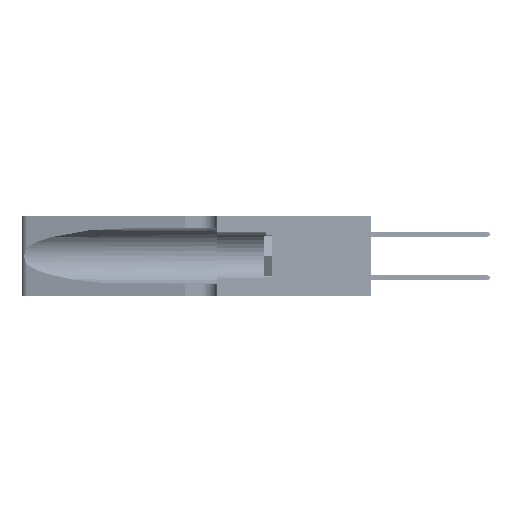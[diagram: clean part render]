
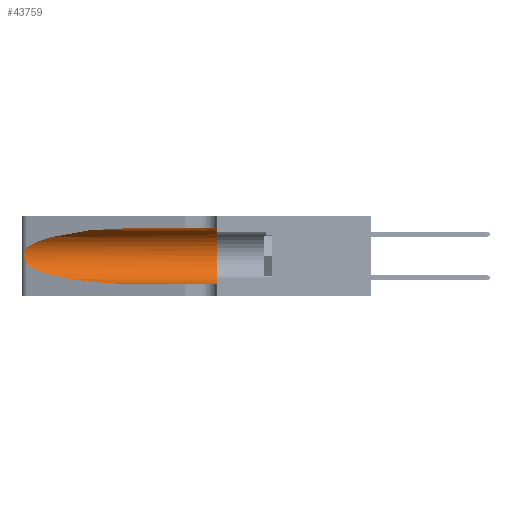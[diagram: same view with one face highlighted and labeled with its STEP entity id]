
A CAD part, left-side view. The second image highlights one B-rep face of the part: STEP entity #43759.
In plain terms, the highlighted cylindrical face has radius 3.308 mm (diameter 6.617 mm), a partial arc.
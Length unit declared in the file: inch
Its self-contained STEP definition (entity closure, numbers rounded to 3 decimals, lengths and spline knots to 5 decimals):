
#577 = CARTESIAN_POINT ( 'NONE',  ( 0.1305, 0.72297, 0.31525 ) ) ;
#794 = CARTESIAN_POINT ( 'NONE',  ( 0.25487, 1.22718, 0.22369 ) ) ;
#3253 = CARTESIAN_POINT ( 'NONE',  ( 0.18966, 0.96281, 0.31525 ) ) ;
#4161 = LINE ( 'NONE', #14341, #13640 ) ;
#4874 = CARTESIAN_POINT ( 'NONE',  ( 0.25854, 1.2359, 0.20912 ) ) ;
#5238 = ORIENTED_EDGE ( 'NONE', *, *, #36718, .T. ) ;
#5308 = ORIENTED_EDGE ( 'NONE', *, *, #21669, .T. ) ;
#6125 = DIRECTION ( 'NONE',  ( 0., -1., 0. ) ) ;
#7294 = CARTESIAN_POINT ( 'NONE',  ( 0.2373, 1.15595, 0.28018 ) ) ;
#8201 = VECTOR ( 'NONE', #6125, 39.37008 ) ;
#8937 = CARTESIAN_POINT ( 'NONE',  ( 0.26075, 1.23896, 0.19203 ) ) ;
#9291 = CARTESIAN_POINT ( 'NONE',  ( 0.25487, 1.22718, 0.22369 ) ) ;
#10169 = CARTESIAN_POINT ( 'NONE',  ( 0.1305, 1.61858, 0.185 ) ) ;
#11039 = EDGE_CURVE ( 'NONE', #23469, #43765, #18882, .T. ) ;
#12251 = DIRECTION ( 'NONE',  ( 0., 1., 0. ) ) ;
#12775 =( BOUNDED_CURVE ( )  B_SPLINE_CURVE ( 3, ( #29696, #41445, #13868, #41618 ),
 .UNSPECIFIED., .F., .F. ) 
 B_SPLINE_CURVE_WITH_KNOTS ( ( 4, 4 ),
 ( 3.44316, 4.71239 ),
 .UNSPECIFIED. ) 
 CURVE ( )  GEOMETRIC_REPRESENTATION_ITEM ( )  RATIONAL_B_SPLINE_CURVE ( ( 1., 0.87, 0.87, 1. ) ) 
 REPRESENTATION_ITEM ( '' )  );
#12976 = CARTESIAN_POINT ( 'NONE',  ( 0.26017, 1.23833, 0.17102 ) ) ;
#13640 = VECTOR ( 'NONE', #22187, 39.37008 ) ;
#13868 = CARTESIAN_POINT ( 'NONE',  ( 0.18966, 0.96281, 0.05475 ) ) ;
#14341 = CARTESIAN_POINT ( 'NONE',  ( 0.1305, 1.61858, 0.05475 ) ) ;
#15547 = EDGE_CURVE ( 'NONE', #15604, #24148, #22069, .T. ) ;
#15604 = VERTEX_POINT ( 'NONE', #9291 ) ;
#16342 = ORIENTED_EDGE ( 'NONE', *, *, #11039, .F. ) ;
#17000 = CARTESIAN_POINT ( 'NONE',  ( 0.25789, 1.23486, 0.15765 ) ) ;
#17660 = EDGE_CURVE ( 'NONE', #24148, #20449, #12775, .T. ) ;
#18235 =( BOUNDED_CURVE ( )  B_SPLINE_CURVE ( 3, ( #46900, #3253, #7294, #35185 ),
 .UNSPECIFIED., .F., .T. ) 
 B_SPLINE_CURVE_WITH_KNOTS ( ( 4, 4 ),
 ( 1.5708, 2.84003 ),
 .UNSPECIFIED. ) 
 CURVE ( )  GEOMETRIC_REPRESENTATION_ITEM ( )  RATIONAL_B_SPLINE_CURVE ( ( 1., 0.87, 0.87, 1. ) ) 
 REPRESENTATION_ITEM ( '' )  );
#18882 = LINE ( 'NONE', #45776, #8201 ) ;
#20449 = VERTEX_POINT ( 'NONE', #43527 ) ;
#20484 = EDGE_CURVE ( 'NONE', #43765, #50777, #27460, .T. ) ;
#21013 = CARTESIAN_POINT ( 'NONE',  ( 0.25555, 1.22993, 0.14849 ) ) ;
#21669 = EDGE_CURVE ( 'NONE', #20449, #50777, #4161, .T. ) ;
#22069 = B_SPLINE_CURVE_WITH_KNOTS ( 'NONE', 3,
 ( #794, #24819, #44551, #28825, #4874, #32799, #8937, #36760, #12976, #40776, #17000, #44726, #21013, #48666 ),
 .UNSPECIFIED., .F., .F.,
 ( 4, 2, 2, 2, 2, 2, 4 ),
 ( 0., 0.00027, 0.00053, 0.00107, 0.0016, 0.00187, 0.00214 ),
 .UNSPECIFIED. ) ;
#22187 = DIRECTION ( 'NONE',  ( 0., -1., 0. ) ) ;
#23469 = VERTEX_POINT ( 'NONE', #577 ) ;
#24148 = VERTEX_POINT ( 'NONE', #37359 ) ;
#24819 = CARTESIAN_POINT ( 'NONE',  ( 0.25555, 1.22994, 0.2215 ) ) ;
#26205 = DIRECTION ( 'NONE',  ( 0., 0., -1. ) ) ;
#26287 = FACE_OUTER_BOUND ( 'NONE', #33118, .T. ) ;
#26637 = ORIENTED_EDGE ( 'NONE', *, *, #17660, .T. ) ;
#27460 = CIRCLE ( 'NONE', #37682, 0.13025 ) ;
#28825 = CARTESIAN_POINT ( 'NONE',  ( 0.25787, 1.23484, 0.2124 ) ) ;
#29696 = CARTESIAN_POINT ( 'NONE',  ( 0.25487, 1.22718, 0.14631 ) ) ;
#31105 = ORIENTED_EDGE ( 'NONE', *, *, #20484, .F. ) ;
#32799 = CARTESIAN_POINT ( 'NONE',  ( 0.26018, 1.23835, 0.19895 ) ) ;
#33118 = EDGE_LOOP ( 'NONE', ( #5238, #39814, #26637, #5308, #31105, #16342 ) ) ;
#34172 = CARTESIAN_POINT ( 'NONE',  ( 0.1305, 0.35, 0.31525 ) ) ;
#35185 = CARTESIAN_POINT ( 'NONE',  ( 0.25487, 1.22718, 0.22369 ) ) ;
#36050 = CARTESIAN_POINT ( 'NONE',  ( 0.1305, 0.35, 0.185 ) ) ;
#36718 = EDGE_CURVE ( 'NONE', #23469, #15604, #18235, .T. ) ;
#36760 = CARTESIAN_POINT ( 'NONE',  ( 0.26075, 1.23896, 0.178 ) ) ;
#36984 = AXIS2_PLACEMENT_3D ( 'NONE', #10169, #49849, #26205 ) ;
#37359 = CARTESIAN_POINT ( 'NONE',  ( 0.25487, 1.22718, 0.14631 ) ) ;
#37682 = AXIS2_PLACEMENT_3D ( 'NONE', #36050, #12251, #40062 ) ;
#39814 = ORIENTED_EDGE ( 'NONE', *, *, #15547, .T. ) ;
#40062 = DIRECTION ( 'NONE',  ( 0., 0., 1. ) ) ;
#40776 = CARTESIAN_POINT ( 'NONE',  ( 0.25856, 1.23593, 0.16098 ) ) ;
#41445 = CARTESIAN_POINT ( 'NONE',  ( 0.2373, 1.15595, 0.08982 ) ) ;
#41618 = CARTESIAN_POINT ( 'NONE',  ( 0.1305, 0.72297, 0.05475 ) ) ;
#42144 = CARTESIAN_POINT ( 'NONE',  ( 0.1305, 0.35, 0.05475 ) ) ;
#43527 = CARTESIAN_POINT ( 'NONE',  ( 0.1305, 0.72297, 0.05475 ) ) ;
#43759 = ADVANCED_FACE ( 'NONE', ( #26287 ), #44842, .F. ) ;
#43765 = VERTEX_POINT ( 'NONE', #34172 ) ;
#44551 = CARTESIAN_POINT ( 'NONE',  ( 0.25639, 1.23184, 0.21858 ) ) ;
#44726 = CARTESIAN_POINT ( 'NONE',  ( 0.25639, 1.23186, 0.15144 ) ) ;
#44842 = CYLINDRICAL_SURFACE ( 'NONE', #36984, 0.13025 ) ;
#45776 = CARTESIAN_POINT ( 'NONE',  ( 0.1305, 1.61858, 0.31525 ) ) ;
#46900 = CARTESIAN_POINT ( 'NONE',  ( 0.1305, 0.72297, 0.31525 ) ) ;
#48666 = CARTESIAN_POINT ( 'NONE',  ( 0.25487, 1.22718, 0.14631 ) ) ;
#49849 = DIRECTION ( 'NONE',  ( 0., -1., 0. ) ) ;
#50777 = VERTEX_POINT ( 'NONE', #42144 ) ;
